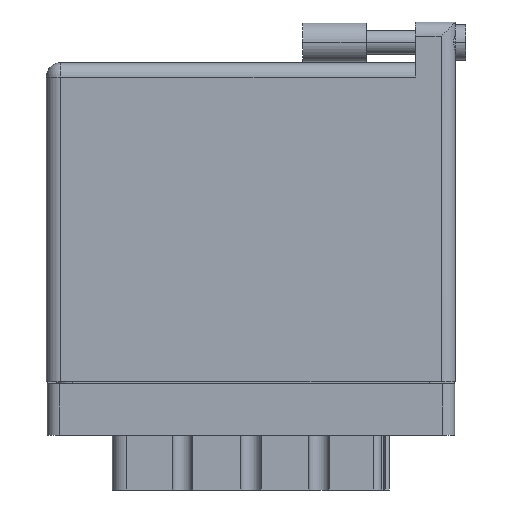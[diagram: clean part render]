
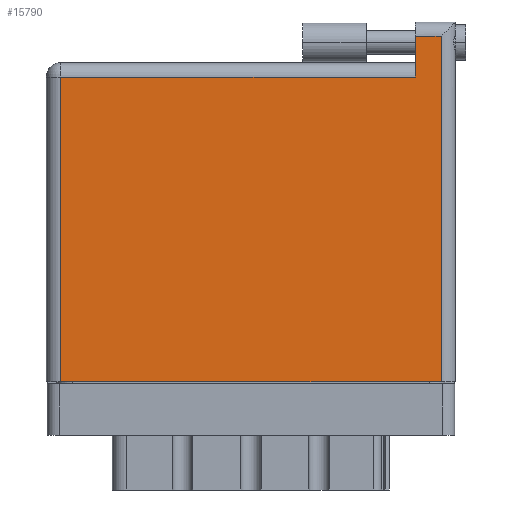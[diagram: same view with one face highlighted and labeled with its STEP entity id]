
A CAD part, front view. The second image highlights one B-rep face of the part: STEP entity #15790.
In plain terms, the highlighted face is planar.
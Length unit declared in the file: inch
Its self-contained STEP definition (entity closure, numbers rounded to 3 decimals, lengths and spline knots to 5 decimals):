
#586 = CARTESIAN_POINT ( 'NONE',  ( 0.07, 1.496, 0. ) ) ;
#1747 = EDGE_CURVE ( 'NONE', #7297, #27444, #7629, .T. ) ;
#3332 = DIRECTION ( 'NONE',  ( 0., 1., 0. ) ) ;
#4539 = CARTESIAN_POINT ( 'NONE',  ( 0.07, 0., 0. ) ) ;
#4705 = ORIENTED_EDGE ( 'NONE', *, *, #31032, .T. ) ;
#4829 = ORIENTED_EDGE ( 'NONE', *, *, #19619, .T. ) ;
#6089 = ORIENTED_EDGE ( 'NONE', *, *, #7012, .T. ) ;
#7012 = EDGE_CURVE ( 'NONE', #36671, #25075, #17749, .T. ) ;
#7297 = VERTEX_POINT ( 'NONE', #19626 ) ;
#7629 = LINE ( 'NONE', #18594, #31845 ) ;
#8222 = VECTOR ( 'NONE', #33017, 39.37008 ) ;
#9371 = CARTESIAN_POINT ( 'NONE',  ( 0.07, 0., 0. ) ) ;
#10782 = CARTESIAN_POINT ( 'NONE',  ( 0., 0., 0. ) ) ;
#12452 = EDGE_CURVE ( 'NONE', #37713, #7297, #37401, .T. ) ;
#14534 = DIRECTION ( 'NONE',  ( 0., -1., 0. ) ) ;
#15134 = EDGE_CURVE ( 'NONE', #27444, #36671, #40151, .T. ) ;
#15790 = ADVANCED_FACE ( 'NONE', ( #30740 ), #39370, .F. ) ;
#15837 = ORIENTED_EDGE ( 'NONE', *, *, #15134, .T. ) ;
#17256 = DIRECTION ( 'NONE',  ( 0., -1., 0. ) ) ;
#17689 = CARTESIAN_POINT ( 'NONE',  ( 1.811, 1.766, 0. ) ) ;
#17749 = LINE ( 'NONE', #32233, #28126 ) ;
#18594 = CARTESIAN_POINT ( 'NONE',  ( 0., 1.696, 0. ) ) ;
#19619 = EDGE_CURVE ( 'NONE', #27699, #37713, #33951, .T. ) ;
#19626 = CARTESIAN_POINT ( 'NONE',  ( 1.938, 1.696, 0. ) ) ;
#23874 = CARTESIAN_POINT ( 'NONE',  ( 0., 1.566, 0. ) ) ;
#25043 = VECTOR ( 'NONE', #17256, 39.37008 ) ;
#25075 = VERTEX_POINT ( 'NONE', #586 ) ;
#25490 = ORIENTED_EDGE ( 'NONE', *, *, #1747, .T. ) ;
#25830 = CARTESIAN_POINT ( 'NONE',  ( 1.938, 1.766, 0. ) ) ;
#27323 = DIRECTION ( 'NONE',  ( 0., 0., -1. ) ) ;
#27444 = VERTEX_POINT ( 'NONE', #29983 ) ;
#27682 = EDGE_LOOP ( 'NONE', ( #4829, #40603, #25490, #15837, #6089, #4705 ) ) ;
#27693 = CARTESIAN_POINT ( 'NONE',  ( 1.938, 0., 0. ) ) ;
#27699 = VERTEX_POINT ( 'NONE', #9371 ) ;
#27921 = CARTESIAN_POINT ( 'NONE',  ( 1.811, 1.496, 0. ) ) ;
#28126 = VECTOR ( 'NONE', #29869, 39.37008 ) ;
#28975 = VECTOR ( 'NONE', #3332, 39.37008 ) ;
#29869 = DIRECTION ( 'NONE',  ( -1., 0., 0. ) ) ;
#29983 = CARTESIAN_POINT ( 'NONE',  ( 1.811, 1.696, 0. ) ) ;
#30740 = FACE_OUTER_BOUND ( 'NONE', #27682, .T. ) ;
#31032 = EDGE_CURVE ( 'NONE', #25075, #27699, #31456, .T. ) ;
#31243 = VECTOR ( 'NONE', #14534, 39.37008 ) ;
#31456 = LINE ( 'NONE', #4539, #25043 ) ;
#31845 = VECTOR ( 'NONE', #34077, 39.37008 ) ;
#32233 = CARTESIAN_POINT ( 'NONE',  ( 0., 1.496, 0. ) ) ;
#33017 = DIRECTION ( 'NONE',  ( 1., 0., 0. ) ) ;
#33951 = LINE ( 'NONE', #10782, #8222 ) ;
#34077 = DIRECTION ( 'NONE',  ( -1., 0., 0. ) ) ;
#34913 = AXIS2_PLACEMENT_3D ( 'NONE', #23874, #27323, #37284 ) ;
#36671 = VERTEX_POINT ( 'NONE', #27921 ) ;
#37284 = DIRECTION ( 'NONE',  ( -1., 0., 0. ) ) ;
#37401 = LINE ( 'NONE', #25830, #28975 ) ;
#37713 = VERTEX_POINT ( 'NONE', #27693 ) ;
#39370 = PLANE ( 'NONE',  #34913 ) ;
#40151 = LINE ( 'NONE', #17689, #31243 ) ;
#40603 = ORIENTED_EDGE ( 'NONE', *, *, #12452, .T. ) ;
